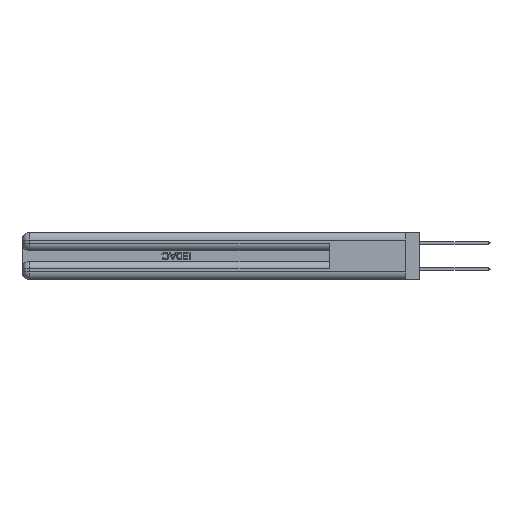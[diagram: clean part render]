
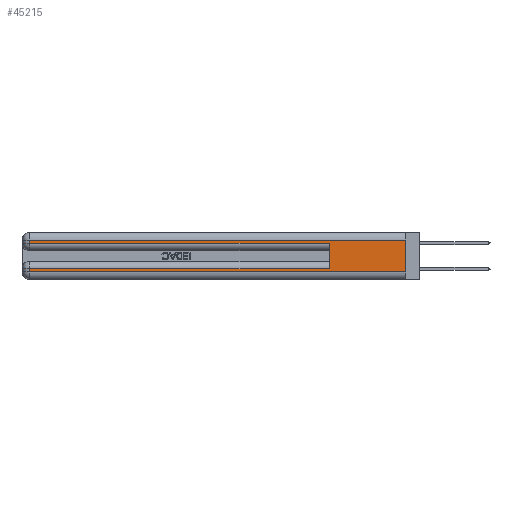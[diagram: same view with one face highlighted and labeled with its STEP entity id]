
A CAD part, left-side view. The second image highlights one B-rep face of the part: STEP entity #45215.
In plain terms, the highlighted planar face has unit normal (-1, 0, 0).
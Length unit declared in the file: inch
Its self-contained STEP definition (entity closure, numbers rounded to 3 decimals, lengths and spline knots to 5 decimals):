
#769 = CARTESIAN_POINT ( 'NONE',  ( 0., 0., 0.37 ) ) ;
#885 = ORIENTED_EDGE ( 'NONE', *, *, #30700, .F. ) ;
#2017 = VERTEX_POINT ( 'NONE', #44064 ) ;
#2652 = CARTESIAN_POINT ( 'NONE',  ( 0., 0., 0.06 ) ) ;
#3041 = EDGE_CURVE ( 'NONE', #26900, #44234, #29243, .T. ) ;
#4006 = DIRECTION ( 'NONE',  ( 1., 0., 0. ) ) ;
#4009 = EDGE_CURVE ( 'NONE', #2017, #44234, #38823, .T. ) ;
#4460 = DIRECTION ( 'NONE',  ( 0., 0., -1. ) ) ;
#4553 = CARTESIAN_POINT ( 'NONE',  ( 0., 2.94, 0.06 ) ) ;
#5275 = FACE_OUTER_BOUND ( 'NONE', #12090, .T. ) ;
#5328 = DIRECTION ( 'NONE',  ( 0., 0., 1. ) ) ;
#5729 = VERTEX_POINT ( 'NONE', #22826 ) ;
#7597 = DIRECTION ( 'NONE',  ( 0., 0., -1. ) ) ;
#7998 = ORIENTED_EDGE ( 'NONE', *, *, #42527, .T. ) ;
#8582 = VECTOR ( 'NONE', #35513, 39.37008 ) ;
#9619 = VECTOR ( 'NONE', #4460, 39.37008 ) ;
#10062 = VECTOR ( 'NONE', #7597, 39.37008 ) ;
#11430 = LINE ( 'NONE', #45544, #41773 ) ;
#12090 = EDGE_LOOP ( 'NONE', ( #39539, #43386, #38008, #28539, #885, #14494, #7998, #12887 ) ) ;
#12568 = CARTESIAN_POINT ( 'NONE',  ( 0., 0.6, 0.145 ) ) ;
#12887 = ORIENTED_EDGE ( 'NONE', *, *, #3041, .T. ) ;
#13703 = CARTESIAN_POINT ( 'NONE',  ( 0., 0.6, 0.285 ) ) ;
#14494 = ORIENTED_EDGE ( 'NONE', *, *, #36952, .T. ) ;
#14571 = EDGE_CURVE ( 'NONE', #2017, #16103, #22292, .T. ) ;
#16103 = VERTEX_POINT ( 'NONE', #18462 ) ;
#16200 = CARTESIAN_POINT ( 'NONE',  ( 0., 0., 0.085 ) ) ;
#16956 = CARTESIAN_POINT ( 'NONE',  ( 0., 0.6, 0.085 ) ) ;
#18462 = CARTESIAN_POINT ( 'NONE',  ( 0., 2.94, 0.31 ) ) ;
#19292 = LINE ( 'NONE', #12568, #29074 ) ;
#19773 = LINE ( 'NONE', #29406, #10062 ) ;
#19869 = DIRECTION ( 'NONE',  ( 0., 1., 0. ) ) ;
#19952 = DIRECTION ( 'NONE',  ( 0., 0., -1. ) ) ;
#22118 = VECTOR ( 'NONE', #19869, 39.37008 ) ;
#22292 = LINE ( 'NONE', #34944, #40597 ) ;
#22601 = EDGE_CURVE ( 'NONE', #16103, #5729, #11430, .T. ) ;
#22826 = CARTESIAN_POINT ( 'NONE',  ( 0., 2.94, 0.285 ) ) ;
#25977 = CARTESIAN_POINT ( 'NONE',  ( 0., 0., 0.37 ) ) ;
#26900 = VERTEX_POINT ( 'NONE', #4553 ) ;
#28539 = ORIENTED_EDGE ( 'NONE', *, *, #28902, .T. ) ;
#28902 = EDGE_CURVE ( 'NONE', #5729, #36470, #45726, .T. ) ;
#29074 = VECTOR ( 'NONE', #5328, 39.37008 ) ;
#29114 = VERTEX_POINT ( 'NONE', #16956 ) ;
#29243 = LINE ( 'NONE', #31839, #8582 ) ;
#29406 = CARTESIAN_POINT ( 'NONE',  ( 0., 2.94, 0.37 ) ) ;
#29661 = DIRECTION ( 'NONE',  ( 0., 0., -1. ) ) ;
#30700 = EDGE_CURVE ( 'NONE', #29114, #36470, #19292, .T. ) ;
#31347 = DIRECTION ( 'NONE',  ( 0., -1., 0. ) ) ;
#31805 = VERTEX_POINT ( 'NONE', #33307 ) ;
#31839 = CARTESIAN_POINT ( 'NONE',  ( 0., 0., 0.06 ) ) ;
#33062 = LINE ( 'NONE', #16200, #22118 ) ;
#33212 = PLANE ( 'NONE',  #35734 ) ;
#33307 = CARTESIAN_POINT ( 'NONE',  ( 0., 2.94, 0.085 ) ) ;
#34944 = CARTESIAN_POINT ( 'NONE',  ( 0., 0., 0.31 ) ) ;
#35028 = CARTESIAN_POINT ( 'NONE',  ( 0., 0., 0.285 ) ) ;
#35513 = DIRECTION ( 'NONE',  ( 0., -1., 0. ) ) ;
#35734 = AXIS2_PLACEMENT_3D ( 'NONE', #25977, #4006, #29661 ) ;
#36470 = VERTEX_POINT ( 'NONE', #13703 ) ;
#36952 = EDGE_CURVE ( 'NONE', #29114, #31805, #33062, .T. ) ;
#38008 = ORIENTED_EDGE ( 'NONE', *, *, #22601, .T. ) ;
#38583 = DIRECTION ( 'NONE',  ( 0., 1., 0. ) ) ;
#38823 = LINE ( 'NONE', #769, #9619 ) ;
#39539 = ORIENTED_EDGE ( 'NONE', *, *, #4009, .F. ) ;
#40597 = VECTOR ( 'NONE', #38583, 39.37008 ) ;
#41773 = VECTOR ( 'NONE', #19952, 39.37008 ) ;
#42527 = EDGE_CURVE ( 'NONE', #31805, #26900, #19773, .T. ) ;
#43386 = ORIENTED_EDGE ( 'NONE', *, *, #14571, .T. ) ;
#44064 = CARTESIAN_POINT ( 'NONE',  ( 0., 0., 0.31 ) ) ;
#44234 = VERTEX_POINT ( 'NONE', #2652 ) ;
#44594 = VECTOR ( 'NONE', #31347, 39.37008 ) ;
#45215 = ADVANCED_FACE ( 'NONE', ( #5275 ), #33212, .F. ) ;
#45544 = CARTESIAN_POINT ( 'NONE',  ( 0., 2.94, 0.37 ) ) ;
#45726 = LINE ( 'NONE', #35028, #44594 ) ;
